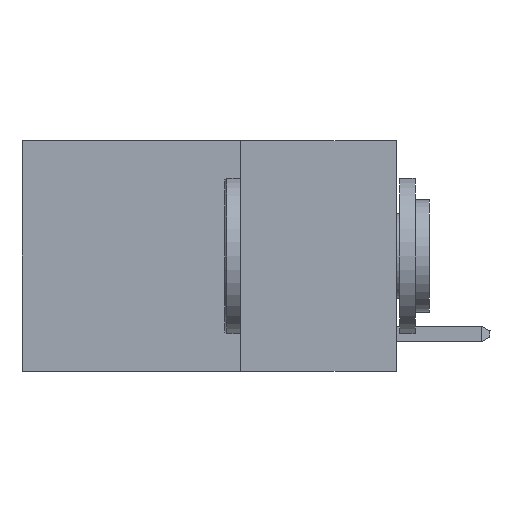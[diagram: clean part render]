
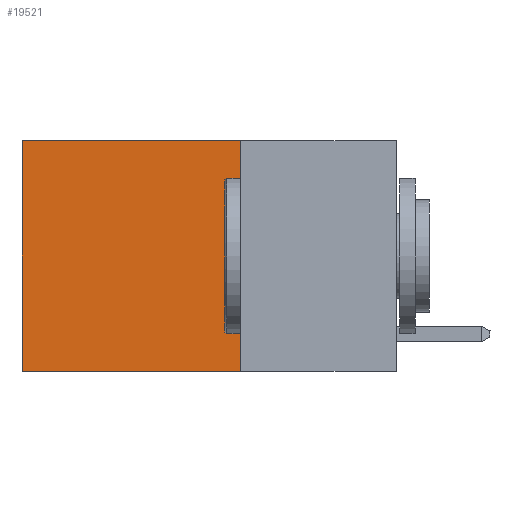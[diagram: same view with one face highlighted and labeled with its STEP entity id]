
A CAD part, left-side view. The second image highlights one B-rep face of the part: STEP entity #19521.
In plain terms, the highlighted planar face has unit normal (-1, 0, 0).
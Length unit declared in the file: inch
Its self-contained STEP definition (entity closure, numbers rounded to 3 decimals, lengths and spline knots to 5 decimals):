
#528 = DIRECTION ( 'NONE',  ( 0., 0., -1. ) ) ;
#1683 = EDGE_CURVE ( 'NONE', #19456, #15243, #2505, .T. ) ;
#2055 = AXIS2_PLACEMENT_3D ( 'NONE', #13210, #13129, #16983 ) ;
#2329 = CARTESIAN_POINT ( 'NONE',  ( 0.2625, 0.6, -0.37 ) ) ;
#2505 = LINE ( 'NONE', #9150, #14091 ) ;
#2907 = DIRECTION ( 'NONE',  ( 0., 1., 0. ) ) ;
#3280 = CARTESIAN_POINT ( 'NONE',  ( 0.2625, 0.25, 0. ) ) ;
#3366 = EDGE_CURVE ( 'NONE', #19456, #21595, #14550, .T. ) ;
#5153 = ORIENTED_EDGE ( 'NONE', *, *, #18404, .T. ) ;
#5877 = FACE_OUTER_BOUND ( 'NONE', #13033, .T. ) ;
#6041 = CARTESIAN_POINT ( 'NONE',  ( 0.2625, 0.25, -0.37 ) ) ;
#8623 = CARTESIAN_POINT ( 'NONE',  ( 0.2625, 0.6, 0. ) ) ;
#8651 = DIRECTION ( 'NONE',  ( 0., 1., 0. ) ) ;
#9150 = CARTESIAN_POINT ( 'NONE',  ( 0.2625, 0.25, 0. ) ) ;
#9864 = PLANE ( 'NONE',  #2055 ) ;
#11524 = CARTESIAN_POINT ( 'NONE',  ( 0.2625, 0.25, -0.37 ) ) ;
#11541 = LINE ( 'NONE', #11524, #15973 ) ;
#11578 = ORIENTED_EDGE ( 'NONE', *, *, #3366, .T. ) ;
#12741 = CARTESIAN_POINT ( 'NONE',  ( 0.2625, 0.25, 0. ) ) ;
#13007 = ORIENTED_EDGE ( 'NONE', *, *, #1683, .F. ) ;
#13033 = EDGE_LOOP ( 'NONE', ( #5153, #13143, #13007, #11578 ) ) ;
#13129 = DIRECTION ( 'NONE',  ( 1., 0., 0. ) ) ;
#13143 = ORIENTED_EDGE ( 'NONE', *, *, #21553, .F. ) ;
#13210 = CARTESIAN_POINT ( 'NONE',  ( 0.2625, 0.25, 0. ) ) ;
#13424 = VECTOR ( 'NONE', #13710, 39.37008 ) ;
#13710 = DIRECTION ( 'NONE',  ( 0., 0., -1. ) ) ;
#14091 = VECTOR ( 'NONE', #528, 39.37008 ) ;
#14550 = LINE ( 'NONE', #3280, #21736 ) ;
#15243 = VERTEX_POINT ( 'NONE', #6041 ) ;
#15353 = LINE ( 'NONE', #8623, #13424 ) ;
#15533 = CARTESIAN_POINT ( 'NONE',  ( 0.2625, 0.6, 0. ) ) ;
#15973 = VECTOR ( 'NONE', #2907, 39.37008 ) ;
#16983 = DIRECTION ( 'NONE',  ( 0., 0., -1. ) ) ;
#18404 = EDGE_CURVE ( 'NONE', #21595, #21908, #15353, .T. ) ;
#19456 = VERTEX_POINT ( 'NONE', #12741 ) ;
#19521 = ADVANCED_FACE ( 'NONE', ( #5877 ), #9864, .F. ) ;
#21553 = EDGE_CURVE ( 'NONE', #15243, #21908, #11541, .T. ) ;
#21595 = VERTEX_POINT ( 'NONE', #15533 ) ;
#21736 = VECTOR ( 'NONE', #8651, 39.37008 ) ;
#21908 = VERTEX_POINT ( 'NONE', #2329 ) ;
